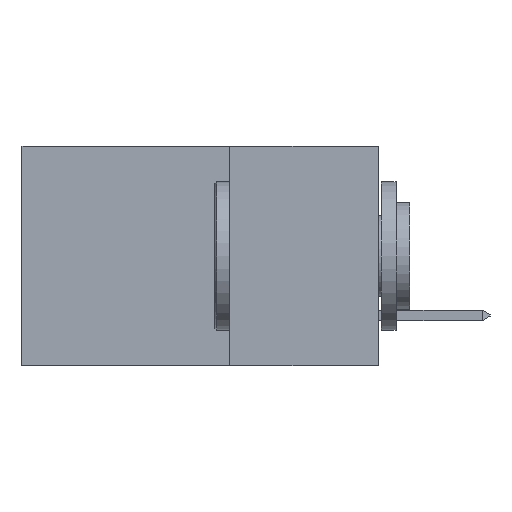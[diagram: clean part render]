
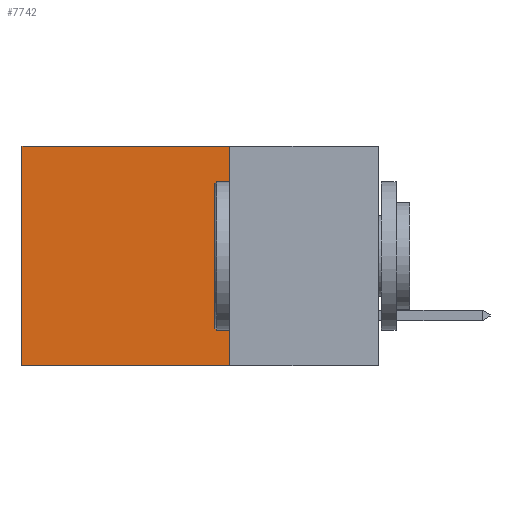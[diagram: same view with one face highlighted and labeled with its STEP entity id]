
A CAD part, left-side view. The second image highlights one B-rep face of the part: STEP entity #7742.
In plain terms, the highlighted planar face has unit normal (-1, 0, 0).
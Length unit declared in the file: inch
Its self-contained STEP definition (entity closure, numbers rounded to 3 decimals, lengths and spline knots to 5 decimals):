
#108 = DIRECTION ( 'NONE',  ( 0., 1., 0. ) ) ;
#265 = CARTESIAN_POINT ( 'NONE',  ( 0.298, 0.25, -0.37 ) ) ;
#1098 = ORIENTED_EDGE ( 'NONE', *, *, #2177, .F. ) ;
#1261 = VECTOR ( 'NONE', #21167, 39.37008 ) ;
#1724 = EDGE_CURVE ( 'NONE', #16164, #4810, #10314, .T. ) ;
#1798 = LINE ( 'NONE', #7556, #1261 ) ;
#2177 = EDGE_CURVE ( 'NONE', #5690, #16164, #12721, .T. ) ;
#2505 = CARTESIAN_POINT ( 'NONE',  ( 0.298, 0.25, 0. ) ) ;
#3565 = CARTESIAN_POINT ( 'NONE',  ( 0.298, 0.25, 0. ) ) ;
#3723 = DIRECTION ( 'NONE',  ( 0., 1., 0. ) ) ;
#3746 = VERTEX_POINT ( 'NONE', #11506 ) ;
#3790 = CARTESIAN_POINT ( 'NONE',  ( 0.298, 0.25, -0.37 ) ) ;
#4810 = VERTEX_POINT ( 'NONE', #20026 ) ;
#4822 = ORIENTED_EDGE ( 'NONE', *, *, #20380, .T. ) ;
#5476 = ORIENTED_EDGE ( 'NONE', *, *, #8404, .T. ) ;
#5690 = VERTEX_POINT ( 'NONE', #2505 ) ;
#7127 = EDGE_LOOP ( 'NONE', ( #4822, #14162, #1098, #5476 ) ) ;
#7556 = CARTESIAN_POINT ( 'NONE',  ( 0.298, 0.6, 0. ) ) ;
#7742 = ADVANCED_FACE ( 'NONE', ( #18816 ), #20132, .F. ) ;
#8404 = EDGE_CURVE ( 'NONE', #5690, #3746, #18537, .T. ) ;
#9226 = VECTOR ( 'NONE', #19222, 39.37008 ) ;
#9246 = VECTOR ( 'NONE', #3723, 39.37008 ) ;
#10297 = AXIS2_PLACEMENT_3D ( 'NONE', #18458, #21752, #11698 ) ;
#10314 = LINE ( 'NONE', #3790, #9246 ) ;
#11506 = CARTESIAN_POINT ( 'NONE',  ( 0.298, 0.6, 0. ) ) ;
#11698 = DIRECTION ( 'NONE',  ( 0., 0., -1. ) ) ;
#12721 = LINE ( 'NONE', #19068, #9226 ) ;
#14071 = VECTOR ( 'NONE', #108, 39.37008 ) ;
#14162 = ORIENTED_EDGE ( 'NONE', *, *, #1724, .F. ) ;
#16164 = VERTEX_POINT ( 'NONE', #265 ) ;
#18458 = CARTESIAN_POINT ( 'NONE',  ( 0.298, 0.25, 0. ) ) ;
#18537 = LINE ( 'NONE', #3565, #14071 ) ;
#18816 = FACE_OUTER_BOUND ( 'NONE', #7127, .T. ) ;
#19068 = CARTESIAN_POINT ( 'NONE',  ( 0.298, 0.25, 0. ) ) ;
#19222 = DIRECTION ( 'NONE',  ( 0., 0., -1. ) ) ;
#20026 = CARTESIAN_POINT ( 'NONE',  ( 0.298, 0.6, -0.37 ) ) ;
#20132 = PLANE ( 'NONE',  #10297 ) ;
#20380 = EDGE_CURVE ( 'NONE', #3746, #4810, #1798, .T. ) ;
#21167 = DIRECTION ( 'NONE',  ( 0., 0., -1. ) ) ;
#21752 = DIRECTION ( 'NONE',  ( 1., 0., 0. ) ) ;
